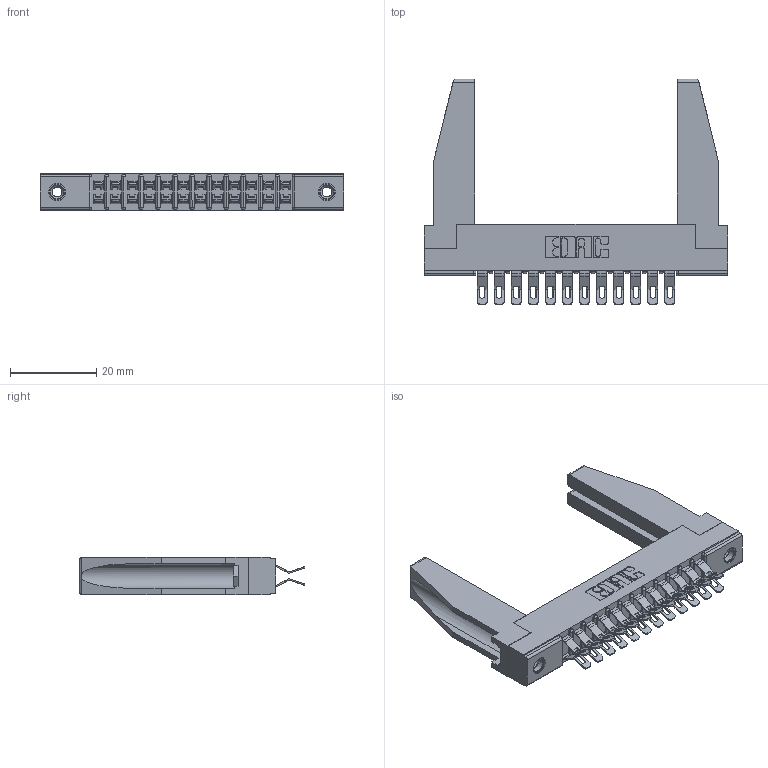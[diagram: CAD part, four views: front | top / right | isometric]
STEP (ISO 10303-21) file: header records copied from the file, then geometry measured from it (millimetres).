
FILE_DESCRIPTION (( 'STEP AP203' ), '1' );
FILE_NAME ('307-024-555-278.STEP', '2019-09-05T22:19:57', ( '' ), ( '' ), 'SwSTEP 2.0', 'SolidWorks 2016', '' );
FILE_SCHEMA (( 'CONFIG_CONTROL_DESIGN' ));
Length unit declared in the file: inch
Products named in the file (5): 307-290-001_555; 345-250-001_345-250-001-102; 307-024-555-278; 307-220-078; 307 Part_.156 Dia Mounting Holes
Assembly tree (29 placements, depth 2):
  307-024-555-278
    307 Part_.156 Dia Mounting Holes
    307-290-001_555  x24
    307-220-078  x2
    345-250-001_345-250-001-102  x2
Bounding box: 70.56 x 52.45 x 8.71 mm (x, y, z)
Volume: 8681.4 mm3; surface area: 11977.8 mm2
Topology: 29 solids, 29 shells, 1725 faces, 4997 edges, 3254 vertices
Faces by surface type: plane 970, cylinder 713, sphere 26, cone 12, torus 4
Entity records: 17346 total; most frequent: CARTESIAN_POINT 2862, ORIENTED_EDGE 2794, DIRECTION 2777, EDGE_CURVE 1397, VECTOR 1051, LINE 1051, VERTEX_POINT 906, AXIS2_PLACEMENT_3D 863
